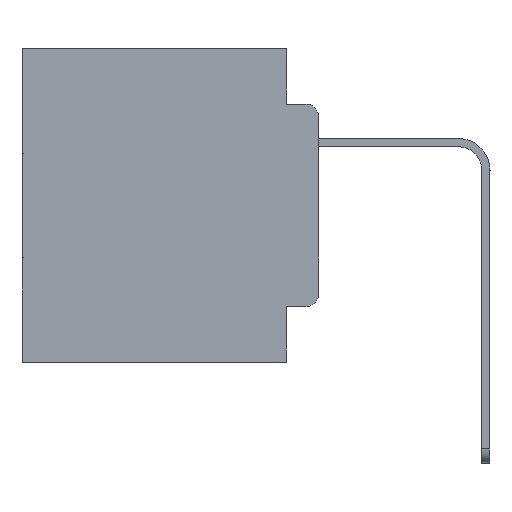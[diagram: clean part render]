
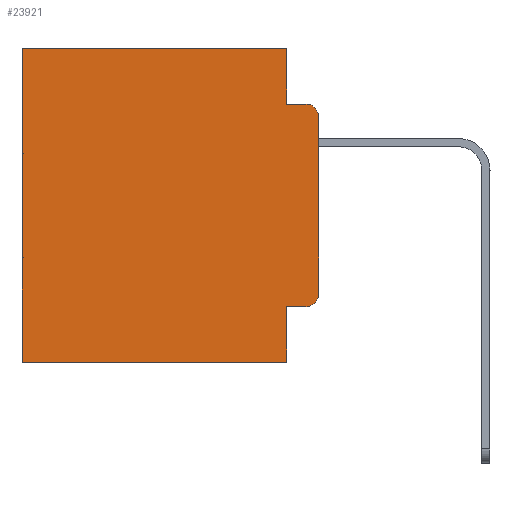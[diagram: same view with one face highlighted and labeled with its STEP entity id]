
A CAD part, left-side view. The second image highlights one B-rep face of the part: STEP entity #23921.
In plain terms, the highlighted planar face has unit normal (-1, 0, 0).
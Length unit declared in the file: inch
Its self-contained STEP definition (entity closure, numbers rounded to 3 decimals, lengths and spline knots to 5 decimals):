
#96 = DIRECTION ( 'NONE',  ( 0., 0., -1. ) ) ;
#107 = DIRECTION ( 'NONE',  ( -1., 0., 0. ) ) ;
#172 = DIRECTION ( 'NONE',  ( 0., 0., -1. ) ) ;
#344 = LINE ( 'NONE', #9941, #10799 ) ;
#709 = VECTOR ( 'NONE', #1216, 39.37008 ) ;
#1000 = LINE ( 'NONE', #22395, #12502 ) ;
#1065 = LINE ( 'NONE', #21709, #709 ) ;
#1216 = DIRECTION ( 'NONE',  ( 0., 1., 0. ) ) ;
#1371 = DIRECTION ( 'NONE',  ( 0., 0., -1. ) ) ;
#1764 = VERTEX_POINT ( 'NONE', #28625 ) ;
#1773 = EDGE_CURVE ( 'NONE', #6554, #15656, #344, .T. ) ;
#3070 = DIRECTION ( 'NONE',  ( 0., -1., 0. ) ) ;
#3404 = CARTESIAN_POINT ( 'NONE',  ( 0.298, 0.051, 0. ) ) ;
#3758 = AXIS2_PLACEMENT_3D ( 'NONE', #10333, #17369, #1371 ) ;
#3818 = LINE ( 'NONE', #13885, #6724 ) ;
#4333 = CARTESIAN_POINT ( 'NONE',  ( 0.298, 0., -0.1085 ) ) ;
#5221 = ORIENTED_EDGE ( 'NONE', *, *, #16925, .F. ) ;
#5650 = DIRECTION ( 'NONE',  ( 0., 1., 0. ) ) ;
#6254 = VERTEX_POINT ( 'NONE', #9912 ) ;
#6554 = VERTEX_POINT ( 'NONE', #6838 ) ;
#6724 = VECTOR ( 'NONE', #96, 39.37008 ) ;
#6786 = DIRECTION ( 'NONE',  ( 0., 0., -1. ) ) ;
#6838 = CARTESIAN_POINT ( 'NONE',  ( 0.298, 0.051, -0.0885 ) ) ;
#6955 = CARTESIAN_POINT ( 'NONE',  ( 0.298, 0.473, 0. ) ) ;
#7127 = FACE_OUTER_BOUND ( 'NONE', #27528, .T. ) ;
#7939 = PLANE ( 'NONE',  #3758 ) ;
#8061 = DIRECTION ( 'NONE',  ( 0., 0., -1. ) ) ;
#8786 = CARTESIAN_POINT ( 'NONE',  ( 0.298, 0.051, 0. ) ) ;
#8844 = CARTESIAN_POINT ( 'NONE',  ( 0.298, 0.02, -0.3915 ) ) ;
#9333 = VERTEX_POINT ( 'NONE', #4333 ) ;
#9533 = EDGE_CURVE ( 'NONE', #14674, #25459, #29066, .T. ) ;
#9586 = VERTEX_POINT ( 'NONE', #12125 ) ;
#9912 = CARTESIAN_POINT ( 'NONE',  ( 0.298, 0.051, -0.5 ) ) ;
#9941 = CARTESIAN_POINT ( 'NONE',  ( 0.298, 0.051, -0.0885 ) ) ;
#10333 = CARTESIAN_POINT ( 'NONE',  ( 0.298, 0., 0. ) ) ;
#10397 = EDGE_CURVE ( 'NONE', #6254, #25459, #17449, .T. ) ;
#10558 = CARTESIAN_POINT ( 'NONE',  ( 0.298, 0., -0.5 ) ) ;
#10799 = VECTOR ( 'NONE', #12329, 39.37008 ) ;
#11983 = ORIENTED_EDGE ( 'NONE', *, *, #10397, .F. ) ;
#12125 = CARTESIAN_POINT ( 'NONE',  ( 0.298, 0., -0.3915 ) ) ;
#12187 = EDGE_CURVE ( 'NONE', #29841, #6254, #26402, .T. ) ;
#12248 = AXIS2_PLACEMENT_3D ( 'NONE', #8844, #27129, #22596 ) ;
#12329 = DIRECTION ( 'NONE',  ( 0., -1., 0. ) ) ;
#12502 = VECTOR ( 'NONE', #3070, 39.37008 ) ;
#13885 = CARTESIAN_POINT ( 'NONE',  ( 0.298, 0., 0. ) ) ;
#14592 = ORIENTED_EDGE ( 'NONE', *, *, #21993, .T. ) ;
#14674 = VERTEX_POINT ( 'NONE', #27092 ) ;
#14821 = CARTESIAN_POINT ( 'NONE',  ( 0.298, 0.473, -0.5 ) ) ;
#15300 = VECTOR ( 'NONE', #172, 39.37008 ) ;
#15392 = CARTESIAN_POINT ( 'NONE',  ( 0.298, 0.051, 0. ) ) ;
#15656 = VERTEX_POINT ( 'NONE', #17080 ) ;
#15894 = DIRECTION ( 'NONE',  ( 0., 0., -1. ) ) ;
#16138 = EDGE_CURVE ( 'NONE', #29841, #1764, #1000, .T. ) ;
#16229 = ORIENTED_EDGE ( 'NONE', *, *, #25082, .T. ) ;
#16925 = EDGE_CURVE ( 'NONE', #20032, #6554, #28745, .T. ) ;
#17080 = CARTESIAN_POINT ( 'NONE',  ( 0.298, 0.02, -0.0885 ) ) ;
#17369 = DIRECTION ( 'NONE',  ( 1., 0., 0. ) ) ;
#17449 = LINE ( 'NONE', #10558, #29428 ) ;
#18224 = VECTOR ( 'NONE', #15894, 39.37008 ) ;
#19652 = ORIENTED_EDGE ( 'NONE', *, *, #9533, .T. ) ;
#20032 = VERTEX_POINT ( 'NONE', #15392 ) ;
#20240 = ORIENTED_EDGE ( 'NONE', *, *, #1773, .F. ) ;
#20401 = CIRCLE ( 'NONE', #12248, 0.02 ) ;
#21709 = CARTESIAN_POINT ( 'NONE',  ( 0.298, 0., 0. ) ) ;
#21993 = EDGE_CURVE ( 'NONE', #20032, #14674, #1065, .T. ) ;
#22395 = CARTESIAN_POINT ( 'NONE',  ( 0.298, 0.051, -0.4115 ) ) ;
#22596 = DIRECTION ( 'NONE',  ( 0., 0., -1. ) ) ;
#22997 = EDGE_CURVE ( 'NONE', #9333, #15656, #26646, .T. ) ;
#23921 = ADVANCED_FACE ( 'NONE', ( #7127 ), #7939, .F. ) ;
#24706 = ORIENTED_EDGE ( 'NONE', *, *, #22997, .T. ) ;
#25082 = EDGE_CURVE ( 'NONE', #1764, #9586, #20401, .T. ) ;
#25268 = ORIENTED_EDGE ( 'NONE', *, *, #16138, .T. ) ;
#25459 = VERTEX_POINT ( 'NONE', #14821 ) ;
#26402 = LINE ( 'NONE', #3404, #28228 ) ;
#26646 = CIRCLE ( 'NONE', #29860, 0.02 ) ;
#27092 = CARTESIAN_POINT ( 'NONE',  ( 0.298, 0.473, 0. ) ) ;
#27129 = DIRECTION ( 'NONE',  ( -1., 0., 0. ) ) ;
#27528 = EDGE_LOOP ( 'NONE', ( #27961, #24706, #20240, #5221, #14592, #19652, #11983, #27629, #25268, #16229 ) ) ;
#27629 = ORIENTED_EDGE ( 'NONE', *, *, #12187, .F. ) ;
#27961 = ORIENTED_EDGE ( 'NONE', *, *, #29566, .F. ) ;
#28228 = VECTOR ( 'NONE', #8061, 39.37008 ) ;
#28625 = CARTESIAN_POINT ( 'NONE',  ( 0.298, 0.02, -0.4115 ) ) ;
#28651 = CARTESIAN_POINT ( 'NONE',  ( 0.298, 0.051, -0.4115 ) ) ;
#28745 = LINE ( 'NONE', #8786, #18224 ) ;
#29066 = LINE ( 'NONE', #6955, #15300 ) ;
#29428 = VECTOR ( 'NONE', #5650, 39.37008 ) ;
#29566 = EDGE_CURVE ( 'NONE', #9333, #9586, #3818, .T. ) ;
#29841 = VERTEX_POINT ( 'NONE', #28651 ) ;
#29860 = AXIS2_PLACEMENT_3D ( 'NONE', #29905, #107, #6786 ) ;
#29905 = CARTESIAN_POINT ( 'NONE',  ( 0.298, 0.02, -0.1085 ) ) ;
